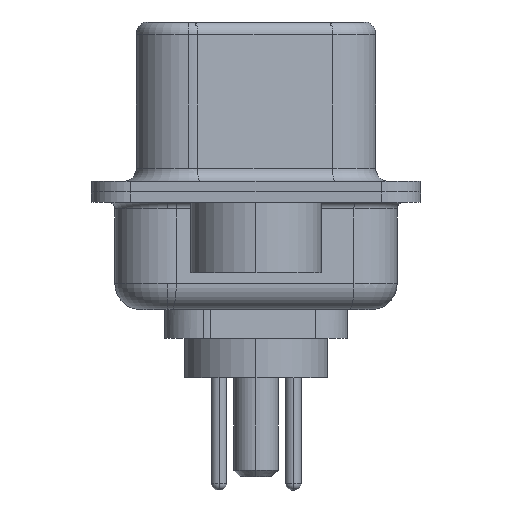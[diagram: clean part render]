
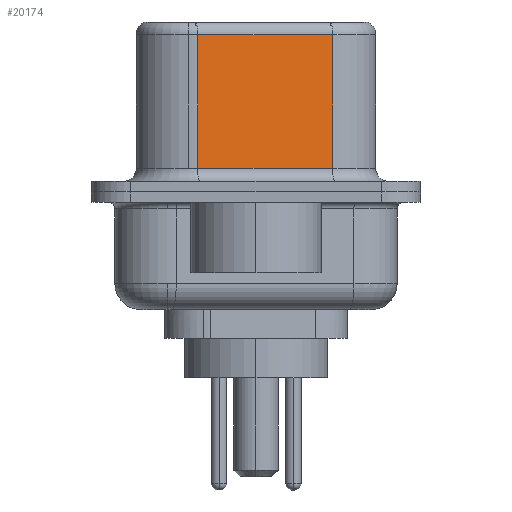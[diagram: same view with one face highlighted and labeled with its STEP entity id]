
A CAD part, left-side view. The second image highlights one B-rep face of the part: STEP entity #20174.
In plain terms, the highlighted planar face has unit normal (-0.985, -0.174, 0).
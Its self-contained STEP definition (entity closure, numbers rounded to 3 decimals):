
#1094 = EDGE_CURVE ( 'NONE', #7350, #3986, #6655, .T. ) ;
#1244 = ORIENTED_EDGE ( 'NONE', *, *, #6908, .T. ) ;
#1345 = DIRECTION ( 'NONE',  ( 0.985, 0.174, 0. ) ) ;
#1488 = LINE ( 'NONE', #7257, #18929 ) ;
#2652 = CARTESIAN_POINT ( 'NONE',  ( 3.67, 2.233, 6.02 ) ) ;
#2871 = VERTEX_POINT ( 'NONE', #17503 ) ;
#2980 = DIRECTION ( 'NONE',  ( 0.174, -0.985, 0. ) ) ;
#3986 = VERTEX_POINT ( 'NONE', #4963 ) ;
#4085 = FACE_OUTER_BOUND ( 'NONE', #5011, .T. ) ;
#4708 = PLANE ( 'NONE',  #20593 ) ;
#4963 = CARTESIAN_POINT ( 'NONE',  ( 4.58, -2.927, 0.9 ) ) ;
#5011 = EDGE_LOOP ( 'NONE', ( #7909, #1244, #10253, #5105 ) ) ;
#5105 = ORIENTED_EDGE ( 'NONE', *, *, #18100, .T. ) ;
#6506 = CARTESIAN_POINT ( 'NONE',  ( 4.58, -2.927, 6.52 ) ) ;
#6655 = LINE ( 'NONE', #6506, #15002 ) ;
#6908 = EDGE_CURVE ( 'NONE', #7350, #20542, #19583, .T. ) ;
#7257 = CARTESIAN_POINT ( 'NONE',  ( 3.67, 2.233, 6.52 ) ) ;
#7350 = VERTEX_POINT ( 'NONE', #7945 ) ;
#7587 = LINE ( 'NONE', #14699, #15436 ) ;
#7909 = ORIENTED_EDGE ( 'NONE', *, *, #1094, .F. ) ;
#7945 = CARTESIAN_POINT ( 'NONE',  ( 4.58, -2.927, 6.02 ) ) ;
#8096 = CARTESIAN_POINT ( 'NONE',  ( 4.58, -2.927, 6.02 ) ) ;
#8805 = DIRECTION ( 'NONE',  ( 0., 0., -1. ) ) ;
#10253 = ORIENTED_EDGE ( 'NONE', *, *, #10946, .T. ) ;
#10946 = EDGE_CURVE ( 'NONE', #20542, #2871, #1488, .T. ) ;
#11418 = DIRECTION ( 'NONE',  ( -0.174, 0.985, 0. ) ) ;
#11449 = CARTESIAN_POINT ( 'NONE',  ( 4.58, -2.927, 6.52 ) ) ;
#13147 = DIRECTION ( 'NONE',  ( -0.174, 0.985, 0. ) ) ;
#14538 = VECTOR ( 'NONE', #11418, 1000. ) ;
#14699 = CARTESIAN_POINT ( 'NONE',  ( 4.58, -2.927, 0.9 ) ) ;
#15002 = VECTOR ( 'NONE', #8805, 1000. ) ;
#15436 = VECTOR ( 'NONE', #2980, 1000. ) ;
#17503 = CARTESIAN_POINT ( 'NONE',  ( 3.67, 2.233, 0.9 ) ) ;
#18100 = EDGE_CURVE ( 'NONE', #2871, #3986, #7587, .T. ) ;
#18929 = VECTOR ( 'NONE', #18991, 1000. ) ;
#18991 = DIRECTION ( 'NONE',  ( 0., 0., -1. ) ) ;
#19583 = LINE ( 'NONE', #8096, #14538 ) ;
#20174 = ADVANCED_FACE ( 'NONE', ( #4085 ), #4708, .F. ) ;
#20542 = VERTEX_POINT ( 'NONE', #2652 ) ;
#20593 = AXIS2_PLACEMENT_3D ( 'NONE', #11449, #1345, #13147 ) ;
